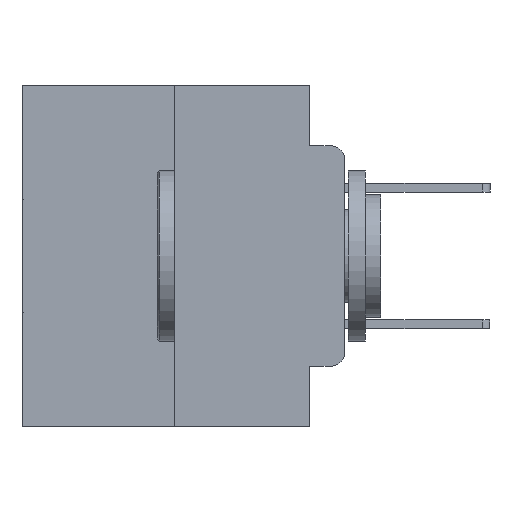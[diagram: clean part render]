
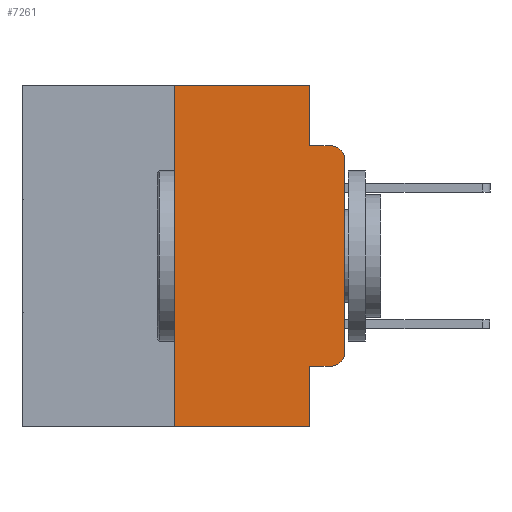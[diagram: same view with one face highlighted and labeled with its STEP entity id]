
A CAD part, left-side view. The second image highlights one B-rep face of the part: STEP entity #7261.
In plain terms, the highlighted planar face has unit normal (-1, 0, 0).
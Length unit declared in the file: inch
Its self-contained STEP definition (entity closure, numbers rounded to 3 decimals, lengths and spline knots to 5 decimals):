
#108 = CARTESIAN_POINT ( 'NONE',  ( 0., 0.25, -0.5 ) ) ;
#679 = ORIENTED_EDGE ( 'NONE', *, *, #17250, .T. ) ;
#1194 = DIRECTION ( 'NONE',  ( -1., 0., 0. ) ) ;
#1302 = EDGE_LOOP ( 'NONE', ( #10054, #12947, #13537, #14595, #14978, #15619, #15707, #15816, #16184, #679 ) ) ;
#2100 = DIRECTION ( 'NONE',  ( 0., 0., -1. ) ) ;
#2726 = AXIS2_PLACEMENT_3D ( 'NONE', #14768, #1194, #16992 ) ;
#3822 = CARTESIAN_POINT ( 'NONE',  ( 0., 0.051, -0.4115 ) ) ;
#4184 = VECTOR ( 'NONE', #25614, 39.37008 ) ;
#4755 = VERTEX_POINT ( 'NONE', #19400 ) ;
#5092 = VERTEX_POINT ( 'NONE', #3822 ) ;
#5598 = CARTESIAN_POINT ( 'NONE',  ( 0., 0.051, -0.4115 ) ) ;
#6597 = CARTESIAN_POINT ( 'NONE',  ( 0., 0.051, 0. ) ) ;
#6805 = PLANE ( 'NONE',  #7191 ) ;
#7191 = AXIS2_PLACEMENT_3D ( 'NONE', #24428, #22329, #9081 ) ;
#7261 = ADVANCED_FACE ( 'NONE', ( #16592 ), #6805, .F. ) ;
#7545 = CARTESIAN_POINT ( 'NONE',  ( 0., 0.051, -0.0885 ) ) ;
#7686 = AXIS2_PLACEMENT_3D ( 'NONE', #26081, #12971, #28247 ) ;
#7718 = DIRECTION ( 'NONE',  ( 0., 0., 1. ) ) ;
#8002 = CIRCLE ( 'NONE', #2726, 0.02 ) ;
#8068 = VECTOR ( 'NONE', #2100, 39.37008 ) ;
#8142 = CARTESIAN_POINT ( 'NONE',  ( 0., 0.051, 0. ) ) ;
#8908 = VERTEX_POINT ( 'NONE', #10618 ) ;
#9081 = DIRECTION ( 'NONE',  ( 0., 0., -1. ) ) ;
#9360 = VERTEX_POINT ( 'NONE', #12145 ) ;
#9435 = LINE ( 'NONE', #9912, #14683 ) ;
#9590 = LINE ( 'NONE', #27575, #25743 ) ;
#9912 = CARTESIAN_POINT ( 'NONE',  ( 0., 0.25, 0. ) ) ;
#10024 = VERTEX_POINT ( 'NONE', #25815 ) ;
#10054 = ORIENTED_EDGE ( 'NONE', *, *, #22237, .T. ) ;
#10219 = LINE ( 'NONE', #23469, #4184 ) ;
#10397 = VECTOR ( 'NONE', #10603, 39.37008 ) ;
#10603 = DIRECTION ( 'NONE',  ( 0., 0., -1. ) ) ;
#10618 = CARTESIAN_POINT ( 'NONE',  ( 0., 0.02, -0.0885 ) ) ;
#11510 = EDGE_CURVE ( 'NONE', #26264, #8908, #13981, .T. ) ;
#12145 = CARTESIAN_POINT ( 'NONE',  ( 0., 0.02, -0.4115 ) ) ;
#12748 = VERTEX_POINT ( 'NONE', #27408 ) ;
#12947 = ORIENTED_EDGE ( 'NONE', *, *, #28545, .T. ) ;
#12971 = DIRECTION ( 'NONE',  ( -1., 0., 0. ) ) ;
#13274 = VECTOR ( 'NONE', #16545, 39.37008 ) ;
#13537 = ORIENTED_EDGE ( 'NONE', *, *, #11510, .F. ) ;
#13981 = LINE ( 'NONE', #23161, #13274 ) ;
#14466 = EDGE_CURVE ( 'NONE', #18889, #10024, #9590, .T. ) ;
#14523 = DIRECTION ( 'NONE',  ( 0., -1., 0. ) ) ;
#14595 = ORIENTED_EDGE ( 'NONE', *, *, #24408, .F. ) ;
#14683 = VECTOR ( 'NONE', #7718, 39.37008 ) ;
#14768 = CARTESIAN_POINT ( 'NONE',  ( 0., 0.02, -0.3915 ) ) ;
#14978 = ORIENTED_EDGE ( 'NONE', *, *, #15818, .F. ) ;
#15619 = ORIENTED_EDGE ( 'NONE', *, *, #22197, .F. ) ;
#15707 = ORIENTED_EDGE ( 'NONE', *, *, #14466, .T. ) ;
#15816 = ORIENTED_EDGE ( 'NONE', *, *, #21364, .F. ) ;
#15818 = EDGE_CURVE ( 'NONE', #12748, #16494, #10219, .T. ) ;
#16184 = ORIENTED_EDGE ( 'NONE', *, *, #27638, .T. ) ;
#16494 = VERTEX_POINT ( 'NONE', #8142 ) ;
#16496 = CARTESIAN_POINT ( 'NONE',  ( 0., 0., -0.1085 ) ) ;
#16545 = DIRECTION ( 'NONE',  ( 0., -1., 0. ) ) ;
#16592 = FACE_OUTER_BOUND ( 'NONE', #1302, .T. ) ;
#16814 = DIRECTION ( 'NONE',  ( 0., 0., 1. ) ) ;
#16992 = DIRECTION ( 'NONE',  ( 0., 0., -1. ) ) ;
#17250 = EDGE_CURVE ( 'NONE', #9360, #4755, #8002, .T. ) ;
#18499 = LINE ( 'NONE', #5598, #24311 ) ;
#18889 = VERTEX_POINT ( 'NONE', #108 ) ;
#18906 = CARTESIAN_POINT ( 'NONE',  ( 0., 0., 0. ) ) ;
#19400 = CARTESIAN_POINT ( 'NONE',  ( 0., 0., -0.3915 ) ) ;
#19874 = LINE ( 'NONE', #6597, #8068 ) ;
#21173 = DIRECTION ( 'NONE',  ( 0., -1., 0. ) ) ;
#21364 = EDGE_CURVE ( 'NONE', #5092, #10024, #19874, .T. ) ;
#22139 = LINE ( 'NONE', #25953, #10397 ) ;
#22197 = EDGE_CURVE ( 'NONE', #18889, #12748, #9435, .T. ) ;
#22237 = EDGE_CURVE ( 'NONE', #4755, #25315, #25592, .T. ) ;
#22329 = DIRECTION ( 'NONE',  ( 1., 0., 0. ) ) ;
#23161 = CARTESIAN_POINT ( 'NONE',  ( 0., 0.051, -0.0885 ) ) ;
#23469 = CARTESIAN_POINT ( 'NONE',  ( 0., 0.473, 0. ) ) ;
#24311 = VECTOR ( 'NONE', #21173, 39.37008 ) ;
#24408 = EDGE_CURVE ( 'NONE', #16494, #26264, #22139, .T. ) ;
#24428 = CARTESIAN_POINT ( 'NONE',  ( 0., 0.473, 0. ) ) ;
#24933 = VECTOR ( 'NONE', #16814, 39.37008 ) ;
#25315 = VERTEX_POINT ( 'NONE', #16496 ) ;
#25592 = LINE ( 'NONE', #18906, #24933 ) ;
#25614 = DIRECTION ( 'NONE',  ( 0., -1., 0. ) ) ;
#25743 = VECTOR ( 'NONE', #14523, 39.37008 ) ;
#25815 = CARTESIAN_POINT ( 'NONE',  ( 0., 0.051, -0.5 ) ) ;
#25953 = CARTESIAN_POINT ( 'NONE',  ( 0., 0.051, 0. ) ) ;
#26081 = CARTESIAN_POINT ( 'NONE',  ( 0., 0.02, -0.1085 ) ) ;
#26264 = VERTEX_POINT ( 'NONE', #7545 ) ;
#27408 = CARTESIAN_POINT ( 'NONE',  ( 0., 0.25, 0. ) ) ;
#27575 = CARTESIAN_POINT ( 'NONE',  ( 0., 0.473, -0.5 ) ) ;
#27638 = EDGE_CURVE ( 'NONE', #5092, #9360, #18499, .T. ) ;
#28247 = DIRECTION ( 'NONE',  ( 0., 0., -1. ) ) ;
#28545 = EDGE_CURVE ( 'NONE', #25315, #8908, #28604, .T. ) ;
#28604 = CIRCLE ( 'NONE', #7686, 0.02 ) ;
